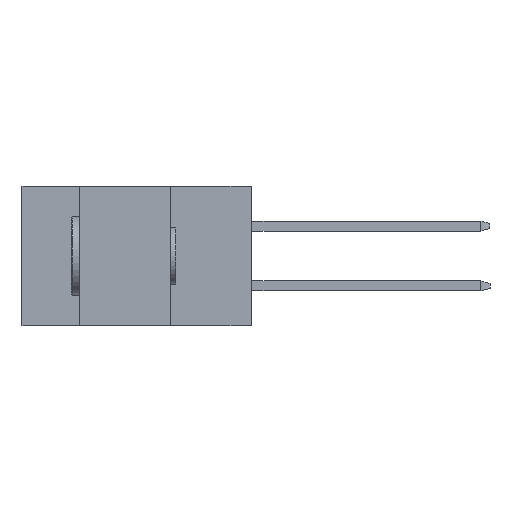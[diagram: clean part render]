
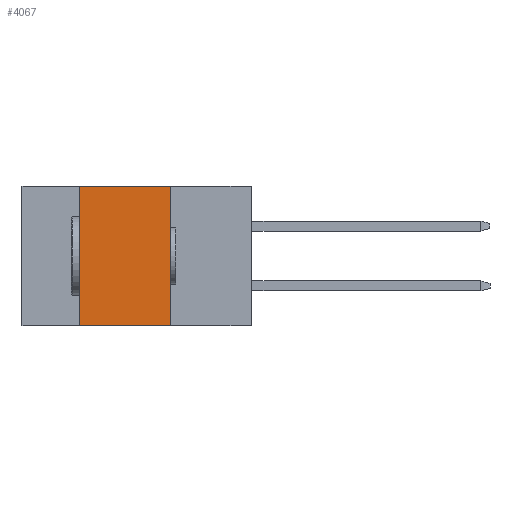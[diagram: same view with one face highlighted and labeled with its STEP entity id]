
A CAD part, left-side view. The second image highlights one B-rep face of the part: STEP entity #4067.
In plain terms, the highlighted planar face has unit normal (-1, 0, 0).
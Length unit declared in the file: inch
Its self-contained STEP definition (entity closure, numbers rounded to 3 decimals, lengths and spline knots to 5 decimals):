
#1402 = ORIENTED_EDGE ( 'NONE', *, *, #11826, .T. ) ;
#1657 = DIRECTION ( 'NONE',  ( 0., -1., 0. ) ) ;
#1999 = VECTOR ( 'NONE', #10096, 39.37008 ) ;
#2435 = CARTESIAN_POINT ( 'NONE',  ( 0., 0.72, 0. ) ) ;
#3028 = LINE ( 'NONE', #20700, #3885 ) ;
#3885 = VECTOR ( 'NONE', #6396, 39.37008 ) ;
#4006 = VERTEX_POINT ( 'NONE', #8162 ) ;
#4067 = ADVANCED_FACE ( 'NONE', ( #7185 ), #13808, .F. ) ;
#4286 = CARTESIAN_POINT ( 'NONE',  ( 0., 0.54, -0.437 ) ) ;
#6395 = LINE ( 'NONE', #11210, #7974 ) ;
#6396 = DIRECTION ( 'NONE',  ( 0., 0., -1. ) ) ;
#6705 = VECTOR ( 'NONE', #14621, 39.37008 ) ;
#7185 = FACE_OUTER_BOUND ( 'NONE', #19934, .T. ) ;
#7188 = EDGE_CURVE ( 'NONE', #12840, #15924, #18076, .T. ) ;
#7389 = ORIENTED_EDGE ( 'NONE', *, *, #9089, .F. ) ;
#7974 = VECTOR ( 'NONE', #1657, 39.37008 ) ;
#8162 = CARTESIAN_POINT ( 'NONE',  ( 0., 0.254, 0. ) ) ;
#9089 = EDGE_CURVE ( 'NONE', #15924, #4006, #13148, .T. ) ;
#10096 = DIRECTION ( 'NONE',  ( 0., 0., 1. ) ) ;
#10188 = CARTESIAN_POINT ( 'NONE',  ( 0., 0.54, -0.437 ) ) ;
#11210 = CARTESIAN_POINT ( 'NONE',  ( 0., 0.72, -0.437 ) ) ;
#11826 = EDGE_CURVE ( 'NONE', #12840, #17702, #6395, .T. ) ;
#12050 = CARTESIAN_POINT ( 'NONE',  ( 0., 0.254, -0.437 ) ) ;
#12840 = VERTEX_POINT ( 'NONE', #4286 ) ;
#13148 = LINE ( 'NONE', #16093, #6705 ) ;
#13808 = PLANE ( 'NONE',  #17336 ) ;
#13963 = ORIENTED_EDGE ( 'NONE', *, *, #17447, .F. ) ;
#14621 = DIRECTION ( 'NONE',  ( 0., -1., 0. ) ) ;
#15924 = VERTEX_POINT ( 'NONE', #16051 ) ;
#16051 = CARTESIAN_POINT ( 'NONE',  ( 0., 0.54, 0. ) ) ;
#16093 = CARTESIAN_POINT ( 'NONE',  ( 0., 0.72, 0. ) ) ;
#16749 = DIRECTION ( 'NONE',  ( 0., 0., -1. ) ) ;
#17336 = AXIS2_PLACEMENT_3D ( 'NONE', #2435, #19926, #16749 ) ;
#17447 = EDGE_CURVE ( 'NONE', #4006, #17702, #3028, .T. ) ;
#17702 = VERTEX_POINT ( 'NONE', #12050 ) ;
#18076 = LINE ( 'NONE', #10188, #1999 ) ;
#19926 = DIRECTION ( 'NONE',  ( 1., 0., 0. ) ) ;
#19934 = EDGE_LOOP ( 'NONE', ( #13963, #7389, #20606, #1402 ) ) ;
#20606 = ORIENTED_EDGE ( 'NONE', *, *, #7188, .F. ) ;
#20700 = CARTESIAN_POINT ( 'NONE',  ( 0., 0.254, -0.437 ) ) ;
